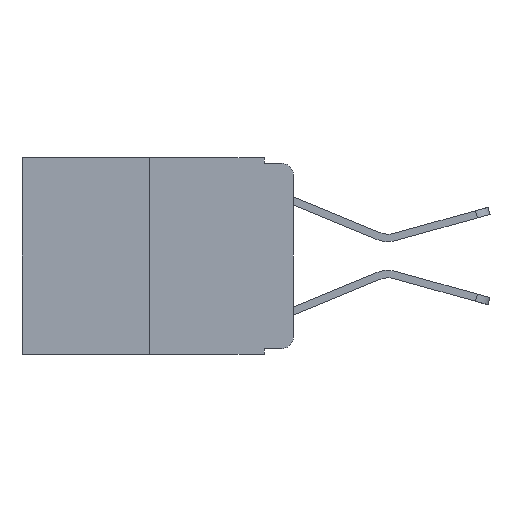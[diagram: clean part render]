
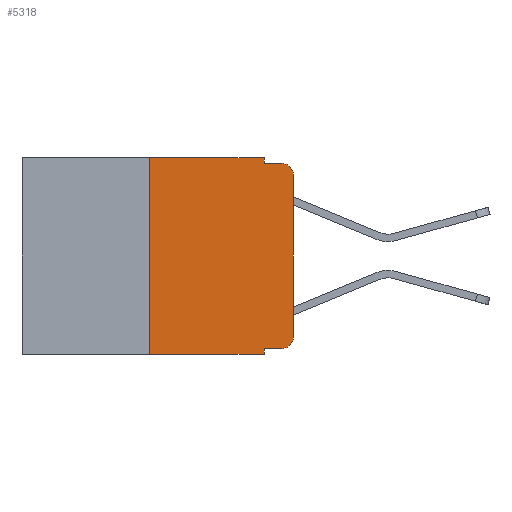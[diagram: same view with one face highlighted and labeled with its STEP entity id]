
A CAD part, left-side view. The second image highlights one B-rep face of the part: STEP entity #5318.
In plain terms, the highlighted planar face has unit normal (-1, 0, 0).
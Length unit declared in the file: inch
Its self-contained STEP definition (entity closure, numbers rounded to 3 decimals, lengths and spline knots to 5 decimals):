
#132 = DIRECTION ( 'NONE',  ( 0., 0., 1. ) ) ;
#183 = VECTOR ( 'NONE', #4136, 39.37008 ) ;
#187 = VECTOR ( 'NONE', #6379, 39.37008 ) ;
#400 = CARTESIAN_POINT ( 'NONE',  ( 0., 0.051, 0. ) ) ;
#662 = DIRECTION ( 'NONE',  ( 1., 0., 0. ) ) ;
#701 = ORIENTED_EDGE ( 'NONE', *, *, #6955, .T. ) ;
#799 = ORIENTED_EDGE ( 'NONE', *, *, #7987, .T. ) ;
#888 = DIRECTION ( 'NONE',  ( 0., -1., 0. ) ) ;
#957 = CARTESIAN_POINT ( 'NONE',  ( 0., 0.02, -0.313 ) ) ;
#1009 = DIRECTION ( 'NONE',  ( -1., 0., 0. ) ) ;
#1075 = VERTEX_POINT ( 'NONE', #8225 ) ;
#1359 = LINE ( 'NONE', #2943, #9812 ) ;
#1467 = CARTESIAN_POINT ( 'NONE',  ( 0., 0.051, -0.333 ) ) ;
#1474 = VERTEX_POINT ( 'NONE', #4315 ) ;
#1817 = ORIENTED_EDGE ( 'NONE', *, *, #6984, .F. ) ;
#1860 = DIRECTION ( 'NONE',  ( 0., 0., -1. ) ) ;
#2363 = DIRECTION ( 'NONE',  ( 0., -1., 0. ) ) ;
#2438 = VERTEX_POINT ( 'NONE', #5448 ) ;
#2489 = CARTESIAN_POINT ( 'NONE',  ( 0., 0.051, 0. ) ) ;
#2524 = CARTESIAN_POINT ( 'NONE',  ( 0., 0.051, -0.343 ) ) ;
#2567 = VERTEX_POINT ( 'NONE', #9751 ) ;
#2737 = CIRCLE ( 'NONE', #9694, 0.02 ) ;
#2774 = ORIENTED_EDGE ( 'NONE', *, *, #6941, .T. ) ;
#2918 = AXIS2_PLACEMENT_3D ( 'NONE', #5741, #662, #5274 ) ;
#2943 = CARTESIAN_POINT ( 'NONE',  ( 0., 0.473, -0.343 ) ) ;
#3047 = ORIENTED_EDGE ( 'NONE', *, *, #7831, .F. ) ;
#3066 = FACE_OUTER_BOUND ( 'NONE', #5659, .T. ) ;
#3680 = VERTEX_POINT ( 'NONE', #2524 ) ;
#4136 = DIRECTION ( 'NONE',  ( 0., 0., -1. ) ) ;
#4315 = CARTESIAN_POINT ( 'NONE',  ( 0., 0.02, -0.333 ) ) ;
#4623 = CARTESIAN_POINT ( 'NONE',  ( 0., 0.051, -0.01 ) ) ;
#5091 = LINE ( 'NONE', #8180, #6888 ) ;
#5274 = DIRECTION ( 'NONE',  ( 0., 0., -1. ) ) ;
#5318 = ADVANCED_FACE ( 'NONE', ( #3066 ), #5757, .F. ) ;
#5448 = CARTESIAN_POINT ( 'NONE',  ( 0., 0.25, -0.343 ) ) ;
#5501 = LINE ( 'NONE', #7177, #187 ) ;
#5659 = EDGE_LOOP ( 'NONE', ( #701, #2774, #10739, #1817, #3047, #9517, #8050, #7504, #7837, #799 ) ) ;
#5681 = VERTEX_POINT ( 'NONE', #2489 ) ;
#5684 = VECTOR ( 'NONE', #888, 39.37008 ) ;
#5741 = CARTESIAN_POINT ( 'NONE',  ( 0., 0.473, 0. ) ) ;
#5757 = PLANE ( 'NONE',  #2918 ) ;
#6228 = VERTEX_POINT ( 'NONE', #10296 ) ;
#6378 = LINE ( 'NONE', #8269, #8212 ) ;
#6379 = DIRECTION ( 'NONE',  ( 0., -1., 0. ) ) ;
#6591 = CARTESIAN_POINT ( 'NONE',  ( 0., 0.051, -0.01 ) ) ;
#6607 = CARTESIAN_POINT ( 'NONE',  ( 0., 0.02, -0.03 ) ) ;
#6733 = LINE ( 'NONE', #1467, #8740 ) ;
#6883 = EDGE_CURVE ( 'NONE', #10627, #6228, #7883, .T. ) ;
#6888 = VECTOR ( 'NONE', #132, 39.37008 ) ;
#6941 = EDGE_CURVE ( 'NONE', #2567, #6228, #2737, .T. ) ;
#6955 = EDGE_CURVE ( 'NONE', #1075, #2567, #5091, .T. ) ;
#6984 = EDGE_CURVE ( 'NONE', #5681, #10627, #8437, .T. ) ;
#7001 = EDGE_CURVE ( 'NONE', #2438, #8058, #6378, .T. ) ;
#7018 = EDGE_CURVE ( 'NONE', #2438, #3680, #1359, .T. ) ;
#7177 = CARTESIAN_POINT ( 'NONE',  ( 0., 0.473, 0. ) ) ;
#7219 = CARTESIAN_POINT ( 'NONE',  ( 0., 0.051, -0.333 ) ) ;
#7380 = DIRECTION ( 'NONE',  ( -1., 0., 0. ) ) ;
#7432 = DIRECTION ( 'NONE',  ( 0., 0., -1. ) ) ;
#7504 = ORIENTED_EDGE ( 'NONE', *, *, #8392, .F. ) ;
#7831 = EDGE_CURVE ( 'NONE', #8058, #5681, #5501, .T. ) ;
#7837 = ORIENTED_EDGE ( 'NONE', *, *, #8504, .T. ) ;
#7883 = LINE ( 'NONE', #4623, #5684 ) ;
#7987 = EDGE_CURVE ( 'NONE', #1474, #1075, #10293, .T. ) ;
#8050 = ORIENTED_EDGE ( 'NONE', *, *, #7018, .T. ) ;
#8058 = VERTEX_POINT ( 'NONE', #10183 ) ;
#8180 = CARTESIAN_POINT ( 'NONE',  ( 0., 0., 0. ) ) ;
#8212 = VECTOR ( 'NONE', #8975, 39.37008 ) ;
#8225 = CARTESIAN_POINT ( 'NONE',  ( 0., 0., -0.313 ) ) ;
#8269 = CARTESIAN_POINT ( 'NONE',  ( 0., 0.25, 0. ) ) ;
#8392 = EDGE_CURVE ( 'NONE', #9314, #3680, #9581, .T. ) ;
#8437 = LINE ( 'NONE', #8947, #8658 ) ;
#8452 = AXIS2_PLACEMENT_3D ( 'NONE', #957, #7380, #1860 ) ;
#8504 = EDGE_CURVE ( 'NONE', #9314, #1474, #6733, .T. ) ;
#8658 = VECTOR ( 'NONE', #9612, 39.37008 ) ;
#8740 = VECTOR ( 'NONE', #2363, 39.37008 ) ;
#8947 = CARTESIAN_POINT ( 'NONE',  ( 0., 0.051, 0. ) ) ;
#8975 = DIRECTION ( 'NONE',  ( 0., 0., 1. ) ) ;
#9314 = VERTEX_POINT ( 'NONE', #7219 ) ;
#9517 = ORIENTED_EDGE ( 'NONE', *, *, #7001, .F. ) ;
#9581 = LINE ( 'NONE', #400, #183 ) ;
#9612 = DIRECTION ( 'NONE',  ( 0., 0., -1. ) ) ;
#9694 = AXIS2_PLACEMENT_3D ( 'NONE', #6607, #1009, #7432 ) ;
#9751 = CARTESIAN_POINT ( 'NONE',  ( 0., 0., -0.03 ) ) ;
#9812 = VECTOR ( 'NONE', #10288, 39.37008 ) ;
#10183 = CARTESIAN_POINT ( 'NONE',  ( 0., 0.25, 0. ) ) ;
#10288 = DIRECTION ( 'NONE',  ( 0., -1., 0. ) ) ;
#10293 = CIRCLE ( 'NONE', #8452, 0.02 ) ;
#10296 = CARTESIAN_POINT ( 'NONE',  ( 0., 0.02, -0.01 ) ) ;
#10627 = VERTEX_POINT ( 'NONE', #6591 ) ;
#10739 = ORIENTED_EDGE ( 'NONE', *, *, #6883, .F. ) ;
